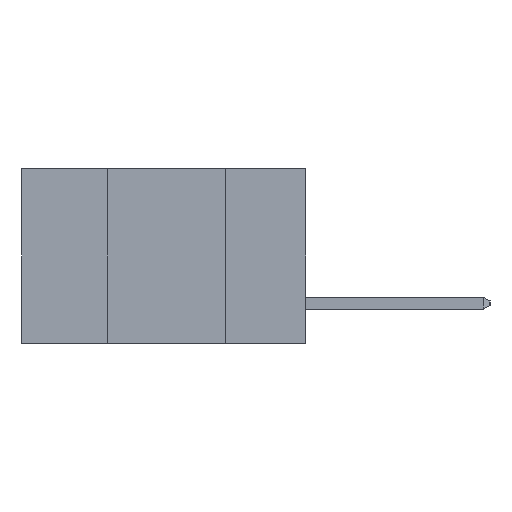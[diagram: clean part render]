
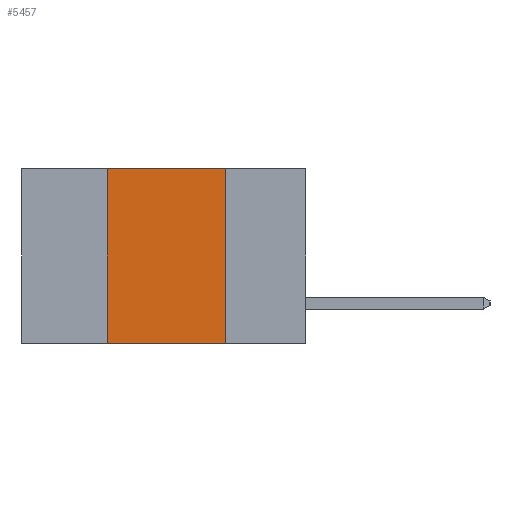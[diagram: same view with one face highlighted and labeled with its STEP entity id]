
A CAD part, left-side view. The second image highlights one B-rep face of the part: STEP entity #5457.
In plain terms, the highlighted planar face has unit normal (-1, 0, 0).
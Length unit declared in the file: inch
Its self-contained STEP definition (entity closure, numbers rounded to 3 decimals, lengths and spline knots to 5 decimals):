
#159 = DIRECTION ( 'NONE',  ( 0., 0., -1. ) ) ;
#174 = DIRECTION ( 'NONE',  ( 1., 0., 0. ) ) ;
#203 = CARTESIAN_POINT ( 'NONE',  ( 0., 0.6, 0. ) ) ;
#246 = PLANE ( 'NONE',  #3960 ) ;
#291 = LINE ( 'NONE', #6525, #10319 ) ;
#423 = ORIENTED_EDGE ( 'NONE', *, *, #6713, .F. ) ;
#557 = LINE ( 'NONE', #12205, #5504 ) ;
#611 = DIRECTION ( 'NONE',  ( 0., -1., 0. ) ) ;
#3960 = AXIS2_PLACEMENT_3D ( 'NONE', #203, #174, #159 ) ;
#4003 = LINE ( 'NONE', #5723, #9087 ) ;
#4698 = EDGE_CURVE ( 'NONE', #4716, #9384, #291, .T. ) ;
#4716 = VERTEX_POINT ( 'NONE', #6159 ) ;
#4907 = CARTESIAN_POINT ( 'NONE',  ( 0., 0.42, -0.37 ) ) ;
#5457 = ADVANCED_FACE ( 'NONE', ( #11072 ), #246, .F. ) ;
#5498 = EDGE_LOOP ( 'NONE', ( #423, #5996, #8509, #11053 ) ) ;
#5504 = VECTOR ( 'NONE', #611, 39.37008 ) ;
#5723 = CARTESIAN_POINT ( 'NONE',  ( 0., 0.17, -0.37 ) ) ;
#5996 = ORIENTED_EDGE ( 'NONE', *, *, #7029, .F. ) ;
#6159 = CARTESIAN_POINT ( 'NONE',  ( 0., 0.42, -0.37 ) ) ;
#6221 = DIRECTION ( 'NONE',  ( 0., -1., 0. ) ) ;
#6525 = CARTESIAN_POINT ( 'NONE',  ( 0., 0.6, -0.37 ) ) ;
#6713 = EDGE_CURVE ( 'NONE', #11795, #9384, #4003, .T. ) ;
#6743 = VECTOR ( 'NONE', #12530, 39.37008 ) ;
#6746 = CARTESIAN_POINT ( 'NONE',  ( 0., 0.42, 0. ) ) ;
#6874 = CARTESIAN_POINT ( 'NONE',  ( 0., 0.17, 0. ) ) ;
#7029 = EDGE_CURVE ( 'NONE', #9734, #11795, #557, .T. ) ;
#7444 = DIRECTION ( 'NONE',  ( 0., 0., -1. ) ) ;
#7501 = CARTESIAN_POINT ( 'NONE',  ( 0., 0.17, -0.37 ) ) ;
#8509 = ORIENTED_EDGE ( 'NONE', *, *, #11078, .F. ) ;
#9087 = VECTOR ( 'NONE', #7444, 39.37008 ) ;
#9384 = VERTEX_POINT ( 'NONE', #7501 ) ;
#9734 = VERTEX_POINT ( 'NONE', #6746 ) ;
#10319 = VECTOR ( 'NONE', #6221, 39.37008 ) ;
#11053 = ORIENTED_EDGE ( 'NONE', *, *, #4698, .T. ) ;
#11072 = FACE_OUTER_BOUND ( 'NONE', #5498, .T. ) ;
#11078 = EDGE_CURVE ( 'NONE', #4716, #9734, #12222, .T. ) ;
#11795 = VERTEX_POINT ( 'NONE', #6874 ) ;
#12205 = CARTESIAN_POINT ( 'NONE',  ( 0., 0.6, 0. ) ) ;
#12222 = LINE ( 'NONE', #4907, #6743 ) ;
#12530 = DIRECTION ( 'NONE',  ( 0., 0., 1. ) ) ;
